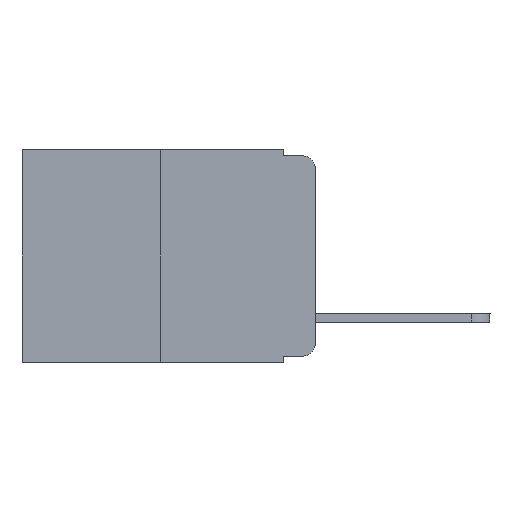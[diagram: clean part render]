
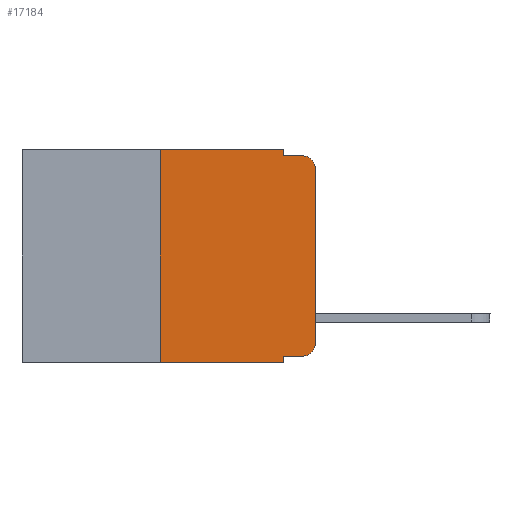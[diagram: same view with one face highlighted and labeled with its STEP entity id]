
A CAD part, left-side view. The second image highlights one B-rep face of the part: STEP entity #17184.
In plain terms, the highlighted planar face has unit normal (-1, 0, 0).
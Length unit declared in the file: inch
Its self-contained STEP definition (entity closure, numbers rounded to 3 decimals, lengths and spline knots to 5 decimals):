
#129 = VERTEX_POINT ( 'NONE', #4733 ) ;
#206 = DIRECTION ( 'NONE',  ( 0., 0., -1. ) ) ;
#311 = CARTESIAN_POINT ( 'NONE',  ( 0., 0.051, -0.01 ) ) ;
#323 = CARTESIAN_POINT ( 'NONE',  ( 0., 0., -0.03 ) ) ;
#361 = VECTOR ( 'NONE', #16593, 39.37008 ) ;
#502 = DIRECTION ( 'NONE',  ( 0., -1., 0. ) ) ;
#594 = CARTESIAN_POINT ( 'NONE',  ( 0., 0.02, -0.03 ) ) ;
#860 = EDGE_CURVE ( 'NONE', #4856, #13439, #5607, .T. ) ;
#1050 = LINE ( 'NONE', #2627, #15324 ) ;
#1241 = CARTESIAN_POINT ( 'NONE',  ( 0., 0.051, -0.333 ) ) ;
#1258 = VECTOR ( 'NONE', #5353, 39.37008 ) ;
#1290 = EDGE_LOOP ( 'NONE', ( #18126, #9758, #9215, #5514, #10478, #9339, #2759, #6823, #17576, #9361 ) ) ;
#1751 = EDGE_CURVE ( 'NONE', #7381, #4856, #8292, .T. ) ;
#2198 = FACE_OUTER_BOUND ( 'NONE', #1290, .T. ) ;
#2213 = CARTESIAN_POINT ( 'NONE',  ( 0., 0.02, -0.333 ) ) ;
#2510 = EDGE_CURVE ( 'NONE', #7109, #12015, #18255, .T. ) ;
#2627 = CARTESIAN_POINT ( 'NONE',  ( 0., 0.25, 0. ) ) ;
#2759 = ORIENTED_EDGE ( 'NONE', *, *, #9402, .T. ) ;
#3266 = LINE ( 'NONE', #1241, #9394 ) ;
#4532 = CARTESIAN_POINT ( 'NONE',  ( 0., 0.473, 0. ) ) ;
#4733 = CARTESIAN_POINT ( 'NONE',  ( 0., 0.25, 0. ) ) ;
#4856 = VERTEX_POINT ( 'NONE', #323 ) ;
#4984 = LINE ( 'NONE', #311, #7723 ) ;
#5136 = CARTESIAN_POINT ( 'NONE',  ( 0., 0.02, -0.01 ) ) ;
#5235 = EDGE_CURVE ( 'NONE', #129, #7109, #16045, .T. ) ;
#5353 = DIRECTION ( 'NONE',  ( 0., 0., -1. ) ) ;
#5514 = ORIENTED_EDGE ( 'NONE', *, *, #2510, .F. ) ;
#5601 = CARTESIAN_POINT ( 'NONE',  ( 0., 0., -0.313 ) ) ;
#5607 = CIRCLE ( 'NONE', #16349, 0.02 ) ;
#6187 = DIRECTION ( 'NONE',  ( -1., 0., 0. ) ) ;
#6823 = ORIENTED_EDGE ( 'NONE', *, *, #7346, .F. ) ;
#7109 = VERTEX_POINT ( 'NONE', #16419 ) ;
#7346 = EDGE_CURVE ( 'NONE', #8181, #14905, #8939, .T. ) ;
#7381 = VERTEX_POINT ( 'NONE', #5601 ) ;
#7490 = CARTESIAN_POINT ( 'NONE',  ( 0., 0.051, -0.333 ) ) ;
#7603 = PLANE ( 'NONE',  #15346 ) ;
#7723 = VECTOR ( 'NONE', #502, 39.37008 ) ;
#7955 = CARTESIAN_POINT ( 'NONE',  ( 0., 0.051, 0. ) ) ;
#8181 = VERTEX_POINT ( 'NONE', #7490 ) ;
#8292 = LINE ( 'NONE', #17635, #12635 ) ;
#8939 = LINE ( 'NONE', #12620, #1258 ) ;
#9035 = DIRECTION ( 'NONE',  ( 0., 0., 1. ) ) ;
#9215 = ORIENTED_EDGE ( 'NONE', *, *, #15071, .F. ) ;
#9218 = VECTOR ( 'NONE', #13156, 39.37008 ) ;
#9339 = ORIENTED_EDGE ( 'NONE', *, *, #12052, .F. ) ;
#9361 = ORIENTED_EDGE ( 'NONE', *, *, #10113, .T. ) ;
#9394 = VECTOR ( 'NONE', #12851, 39.37008 ) ;
#9402 = EDGE_CURVE ( 'NONE', #17745, #14905, #17493, .T. ) ;
#9758 = ORIENTED_EDGE ( 'NONE', *, *, #860, .T. ) ;
#10113 = EDGE_CURVE ( 'NONE', #11233, #7381, #16334, .T. ) ;
#10478 = ORIENTED_EDGE ( 'NONE', *, *, #5235, .F. ) ;
#11233 = VERTEX_POINT ( 'NONE', #2213 ) ;
#11280 = DIRECTION ( 'NONE',  ( -1., 0., 0. ) ) ;
#11974 = DIRECTION ( 'NONE',  ( 0., -1., 0. ) ) ;
#12015 = VERTEX_POINT ( 'NONE', #12787 ) ;
#12052 = EDGE_CURVE ( 'NONE', #17745, #129, #1050, .T. ) ;
#12198 = EDGE_CURVE ( 'NONE', #8181, #11233, #3266, .T. ) ;
#12620 = CARTESIAN_POINT ( 'NONE',  ( 0., 0.051, 0. ) ) ;
#12635 = VECTOR ( 'NONE', #9035, 39.37008 ) ;
#12741 = VECTOR ( 'NONE', #11974, 39.37008 ) ;
#12787 = CARTESIAN_POINT ( 'NONE',  ( 0., 0.051, -0.01 ) ) ;
#12851 = DIRECTION ( 'NONE',  ( 0., -1., 0. ) ) ;
#13156 = DIRECTION ( 'NONE',  ( 0., -1., 0. ) ) ;
#13439 = VERTEX_POINT ( 'NONE', #5136 ) ;
#13442 = DIRECTION ( 'NONE',  ( 0., 0., -1. ) ) ;
#13651 = AXIS2_PLACEMENT_3D ( 'NONE', #17107, #11280, #15591 ) ;
#14022 = CARTESIAN_POINT ( 'NONE',  ( 0., 0.25, -0.343 ) ) ;
#14744 = CARTESIAN_POINT ( 'NONE',  ( 0., 0.051, -0.343 ) ) ;
#14905 = VERTEX_POINT ( 'NONE', #14744 ) ;
#15071 = EDGE_CURVE ( 'NONE', #12015, #13439, #4984, .T. ) ;
#15324 = VECTOR ( 'NONE', #18301, 39.37008 ) ;
#15346 = AXIS2_PLACEMENT_3D ( 'NONE', #4532, #16043, #206 ) ;
#15591 = DIRECTION ( 'NONE',  ( 0., 0., -1. ) ) ;
#16043 = DIRECTION ( 'NONE',  ( 1., 0., 0. ) ) ;
#16045 = LINE ( 'NONE', #17604, #9218 ) ;
#16083 = CARTESIAN_POINT ( 'NONE',  ( 0., 0.473, -0.343 ) ) ;
#16334 = CIRCLE ( 'NONE', #13651, 0.02 ) ;
#16349 = AXIS2_PLACEMENT_3D ( 'NONE', #594, #6187, #13442 ) ;
#16419 = CARTESIAN_POINT ( 'NONE',  ( 0., 0.051, 0. ) ) ;
#16593 = DIRECTION ( 'NONE',  ( 0., 0., -1. ) ) ;
#17107 = CARTESIAN_POINT ( 'NONE',  ( 0., 0.02, -0.313 ) ) ;
#17184 = ADVANCED_FACE ( 'NONE', ( #2198 ), #7603, .F. ) ;
#17493 = LINE ( 'NONE', #16083, #12741 ) ;
#17576 = ORIENTED_EDGE ( 'NONE', *, *, #12198, .T. ) ;
#17604 = CARTESIAN_POINT ( 'NONE',  ( 0., 0.473, 0. ) ) ;
#17635 = CARTESIAN_POINT ( 'NONE',  ( 0., 0., 0. ) ) ;
#17745 = VERTEX_POINT ( 'NONE', #14022 ) ;
#18126 = ORIENTED_EDGE ( 'NONE', *, *, #1751, .T. ) ;
#18255 = LINE ( 'NONE', #7955, #361 ) ;
#18301 = DIRECTION ( 'NONE',  ( 0., 0., 1. ) ) ;
